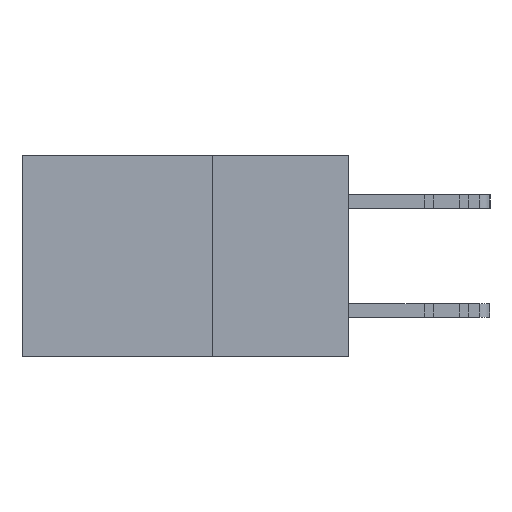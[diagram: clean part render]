
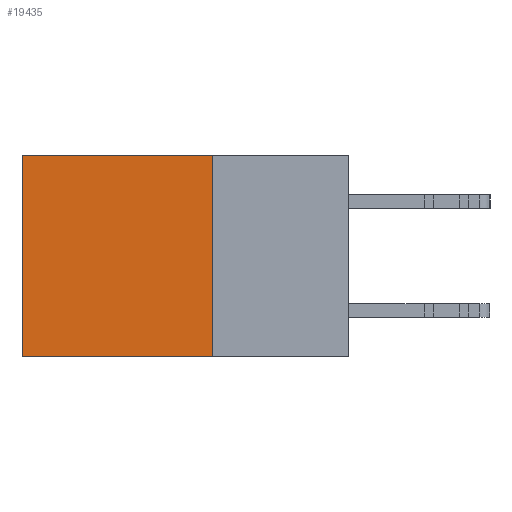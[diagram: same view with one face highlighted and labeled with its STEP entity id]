
A CAD part, left-side view. The second image highlights one B-rep face of the part: STEP entity #19435.
In plain terms, the highlighted planar face has unit normal (-1, 0, 0).
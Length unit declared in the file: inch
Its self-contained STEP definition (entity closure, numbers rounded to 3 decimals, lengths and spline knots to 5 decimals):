
#98 = CARTESIAN_POINT ( 'NONE',  ( 0.2615, 0.25, -0.37 ) ) ;
#342 = LINE ( 'NONE', #2055, #13413 ) ;
#402 = FACE_OUTER_BOUND ( 'NONE', #16408, .T. ) ;
#2055 = CARTESIAN_POINT ( 'NONE',  ( 0.2615, 0.25, -0.37 ) ) ;
#2630 = DIRECTION ( 'NONE',  ( 0., 0., -1. ) ) ;
#3528 = DIRECTION ( 'NONE',  ( 0., 0., -1. ) ) ;
#4518 = VERTEX_POINT ( 'NONE', #18562 ) ;
#5226 = AXIS2_PLACEMENT_3D ( 'NONE', #20607, #24428, #2630 ) ;
#6409 = EDGE_CURVE ( 'NONE', #4518, #22391, #22008, .T. ) ;
#6810 = ORIENTED_EDGE ( 'NONE', *, *, #8385, .T. ) ;
#7399 = CARTESIAN_POINT ( 'NONE',  ( 0.2615, 0.6, -0.37 ) ) ;
#7900 = VERTEX_POINT ( 'NONE', #20951 ) ;
#8385 = EDGE_CURVE ( 'NONE', #7900, #22391, #19911, .T. ) ;
#8626 = VERTEX_POINT ( 'NONE', #19098 ) ;
#9034 = ORIENTED_EDGE ( 'NONE', *, *, #10399, .F. ) ;
#9047 = ORIENTED_EDGE ( 'NONE', *, *, #9129, .T. ) ;
#9097 = DIRECTION ( 'NONE',  ( 0., 1., 0. ) ) ;
#9129 = EDGE_CURVE ( 'NONE', #8626, #7900, #23009, .T. ) ;
#9192 = VECTOR ( 'NONE', #9097, 39.37008 ) ;
#9291 = VECTOR ( 'NONE', #3528, 39.37008 ) ;
#10399 = EDGE_CURVE ( 'NONE', #8626, #4518, #342, .T. ) ;
#11638 = CARTESIAN_POINT ( 'NONE',  ( 0.2615, 0.6, -0.37 ) ) ;
#12604 = PLANE ( 'NONE',  #5226 ) ;
#13413 = VECTOR ( 'NONE', #24374, 39.37008 ) ;
#16408 = EDGE_LOOP ( 'NONE', ( #6810, #19895, #9034, #9047 ) ) ;
#18562 = CARTESIAN_POINT ( 'NONE',  ( 0.2615, 0.25, -0.37 ) ) ;
#19098 = CARTESIAN_POINT ( 'NONE',  ( 0.2615, 0.25, 0. ) ) ;
#19435 = ADVANCED_FACE ( 'NONE', ( #402 ), #12604, .F. ) ;
#19895 = ORIENTED_EDGE ( 'NONE', *, *, #6409, .F. ) ;
#19911 = LINE ( 'NONE', #11638, #9291 ) ;
#20607 = CARTESIAN_POINT ( 'NONE',  ( 0.2615, 0.25, -0.37 ) ) ;
#20951 = CARTESIAN_POINT ( 'NONE',  ( 0.2615, 0.6, 0. ) ) ;
#21032 = CARTESIAN_POINT ( 'NONE',  ( 0.2615, 0.25, 0. ) ) ;
#21176 = VECTOR ( 'NONE', #21883, 39.37008 ) ;
#21883 = DIRECTION ( 'NONE',  ( 0., 1., 0. ) ) ;
#22008 = LINE ( 'NONE', #98, #21176 ) ;
#22391 = VERTEX_POINT ( 'NONE', #7399 ) ;
#23009 = LINE ( 'NONE', #21032, #9192 ) ;
#24374 = DIRECTION ( 'NONE',  ( 0., 0., -1. ) ) ;
#24428 = DIRECTION ( 'NONE',  ( 1., 0., 0. ) ) ;
